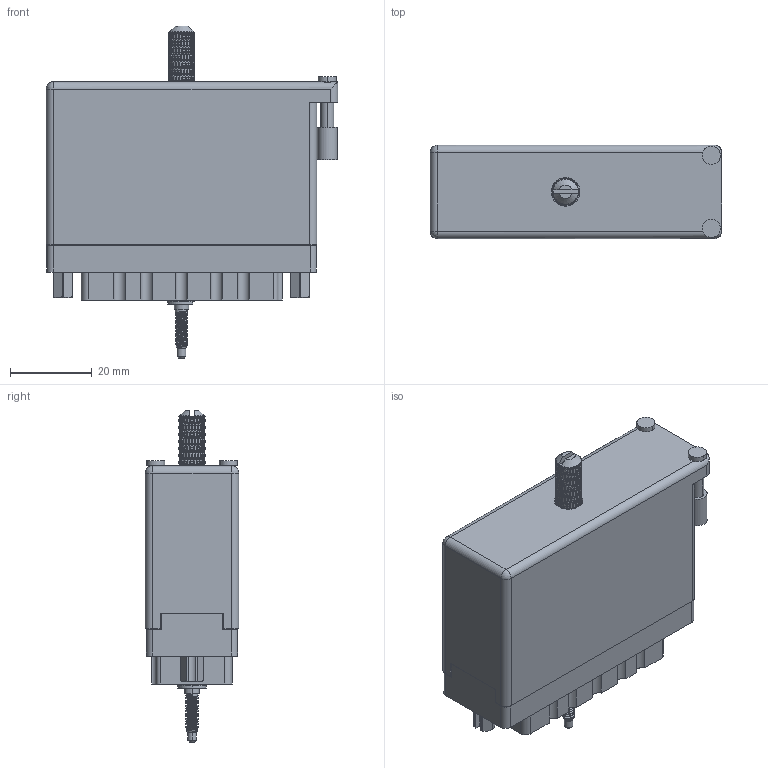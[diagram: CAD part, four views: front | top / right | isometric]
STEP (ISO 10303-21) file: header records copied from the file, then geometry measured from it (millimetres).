
FILE_DESCRIPTION (( 'STEP AP203' ), '1' );
FILE_NAME ('516-056-000-251.STEP', '2020-03-05T19:41:50', ( '' ), ( '' ), 'SwSTEP 2.0', 'SolidWorks 2016', '' );
FILE_SCHEMA (( 'CONFIG_CONTROL_DESIGN' ));
Length unit declared in the file: inch
Products named in the file (11): 516-253-035-100; 516-221-038-102_056; 516-056-000-251; 516-253-138-107; 516-250-038-111; 516-251-035-100; 516-252-021-102_056; 516-230-001_Metal - 056 Side Entry; 516-221-038-102_057; Actuating Screw Assy 038-056; 516 Part Receptacle_056
Assembly tree (12 placements, depth 3):
  516-056-000-251
    516 Part Receptacle_056
    516-230-001_Metal - 056 Side Entry
    516-252-021-102_056  x2
    516-221-038-102_056
    Actuating Screw Assy 038-056
      516-251-035-100
      516-253-035-100  x2
      516-253-138-107
      516-250-038-111
    516-221-038-102_057
Bounding box: 71.12 x 22.83 x 81.03 mm (x, y, z)
Volume: 27151.4 mm3; surface area: 39286.5 mm2
Topology: 11 solids, 11 shells, 2895 faces, 7361 edges, 4504 vertices
Faces by surface type: plane 1049, bspline 1034, cylinder 758, cone 52, sphere 2
Entity records: 120219 total; most frequent: CARTESIAN_POINT 61317, ORIENTED_EDGE 14506, DIRECTION 9410, EDGE_CURVE 7253, VERTEX_POINT 4436, AXIS2_PLACEMENT_3D 3153, VECTOR 3104, LINE 3104
